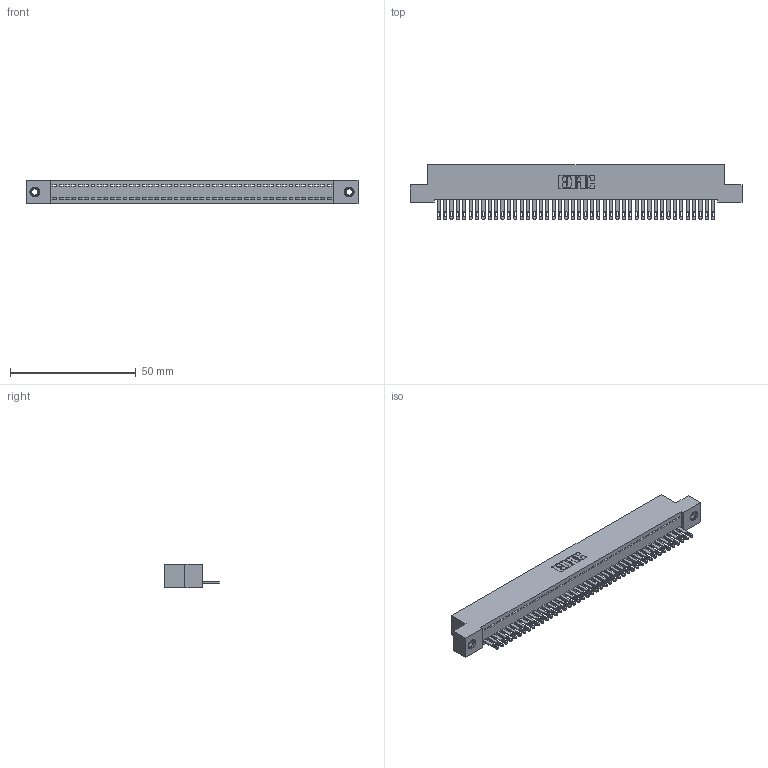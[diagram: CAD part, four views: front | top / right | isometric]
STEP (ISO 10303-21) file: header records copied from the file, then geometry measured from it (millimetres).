
FILE_DESCRIPTION (( 'STEP AP203' ), '1' );
FILE_NAME ('342-044-500-107.STEP', '2019-10-02T18:48:44', ( '' ), ( '' ), 'SwSTEP 2.0', 'SolidWorks 2016', '' );
FILE_SCHEMA (( 'CONFIG_CONTROL_DESIGN' ));
Length unit declared in the file: inch
Products named in the file (4): 345-250-001_345-250-005-103; 342-044-500-107; 342 Part_TI; 345-292-001_345-293-100
Assembly tree (47 placements, depth 2):
  342-044-500-107
    342 Part_TI
    345-292-001_345-293-100  x44
    345-250-001_345-250-005-103  x2
Bounding box: 132.08 x 21.85 x 9.4 mm (x, y, z)
Volume: 11602.7 mm3; surface area: 17194.2 mm2
Topology: 47 solids, 47 shells, 2546 faces, 7827 edges, 5210 vertices
Faces by surface type: plane 1682, cylinder 848, cone 12, torus 4
Entity records: 27624 total; most frequent: CARTESIAN_POINT 4745, ORIENTED_EDGE 4718, DIRECTION 4033, EDGE_CURVE 2359, VECTOR 2207, LINE 2207, VERTEX_POINT 1568, AXIS2_PLACEMENT_3D 913
